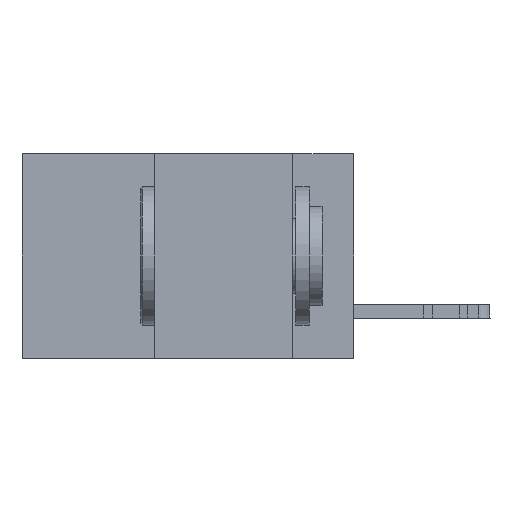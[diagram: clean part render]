
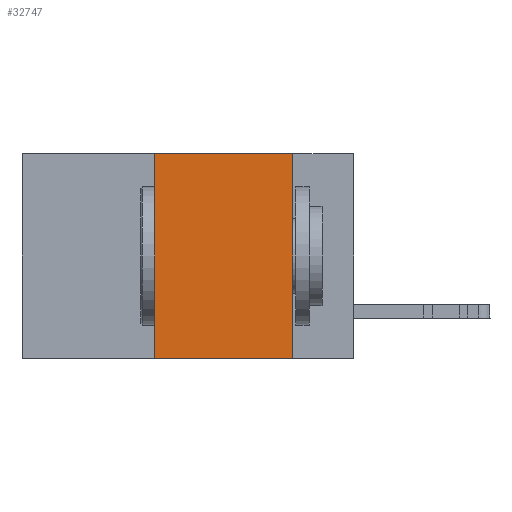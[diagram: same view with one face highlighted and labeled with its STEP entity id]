
A CAD part, left-side view. The second image highlights one B-rep face of the part: STEP entity #32747.
In plain terms, the highlighted planar face has unit normal (-1, 0, 0).
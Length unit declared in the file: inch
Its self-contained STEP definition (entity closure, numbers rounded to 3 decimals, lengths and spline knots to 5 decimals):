
#1204 = VERTEX_POINT ( 'NONE', #24172 ) ;
#1741 = VECTOR ( 'NONE', #41531, 39.37008 ) ;
#6698 = CARTESIAN_POINT ( 'NONE',  ( 0., 0.11, 0. ) ) ;
#12071 = LINE ( 'NONE', #14027, #20456 ) ;
#13984 = FACE_OUTER_BOUND ( 'NONE', #40193, .T. ) ;
#13990 = DIRECTION ( 'NONE',  ( 0., 0., -1. ) ) ;
#14027 = CARTESIAN_POINT ( 'NONE',  ( 0., 0.6, -0.37 ) ) ;
#15195 = VERTEX_POINT ( 'NONE', #22271 ) ;
#15994 = EDGE_CURVE ( 'NONE', #1204, #47161, #20562, .T. ) ;
#16484 = CARTESIAN_POINT ( 'NONE',  ( 0., 0.6, 0. ) ) ;
#17156 = EDGE_CURVE ( 'NONE', #47161, #15195, #27197, .T. ) ;
#18079 = VECTOR ( 'NONE', #13990, 39.37008 ) ;
#19020 = DIRECTION ( 'NONE',  ( 1., 0., 0. ) ) ;
#19328 = CARTESIAN_POINT ( 'NONE',  ( 0., 0.6, 0. ) ) ;
#20456 = VECTOR ( 'NONE', #33123, 39.37008 ) ;
#20562 = LINE ( 'NONE', #16484, #47250 ) ;
#20992 = CARTESIAN_POINT ( 'NONE',  ( 0., 0.11, 0. ) ) ;
#22271 = CARTESIAN_POINT ( 'NONE',  ( 0., 0.11, -0.37 ) ) ;
#23667 = PLANE ( 'NONE',  #24256 ) ;
#24110 = ORIENTED_EDGE ( 'NONE', *, *, #15994, .F. ) ;
#24172 = CARTESIAN_POINT ( 'NONE',  ( 0., 0.36, 0. ) ) ;
#24253 = CARTESIAN_POINT ( 'NONE',  ( 0., 0.36, -0.37 ) ) ;
#24256 = AXIS2_PLACEMENT_3D ( 'NONE', #19328, #19020, #30412 ) ;
#24885 = LINE ( 'NONE', #37453, #1741 ) ;
#25823 = ORIENTED_EDGE ( 'NONE', *, *, #27186, .T. ) ;
#26753 = VERTEX_POINT ( 'NONE', #24253 ) ;
#27186 = EDGE_CURVE ( 'NONE', #26753, #15195, #12071, .T. ) ;
#27197 = LINE ( 'NONE', #6698, #18079 ) ;
#27892 = ORIENTED_EDGE ( 'NONE', *, *, #46252, .F. ) ;
#30412 = DIRECTION ( 'NONE',  ( 0., 0., -1. ) ) ;
#32747 = ADVANCED_FACE ( 'NONE', ( #13984 ), #23667, .F. ) ;
#33123 = DIRECTION ( 'NONE',  ( 0., -1., 0. ) ) ;
#37453 = CARTESIAN_POINT ( 'NONE',  ( 0., 0.36, 0. ) ) ;
#40193 = EDGE_LOOP ( 'NONE', ( #49397, #24110, #27892, #25823 ) ) ;
#41531 = DIRECTION ( 'NONE',  ( 0., 0., 1. ) ) ;
#43512 = DIRECTION ( 'NONE',  ( 0., -1., 0. ) ) ;
#46252 = EDGE_CURVE ( 'NONE', #26753, #1204, #24885, .T. ) ;
#47161 = VERTEX_POINT ( 'NONE', #20992 ) ;
#47250 = VECTOR ( 'NONE', #43512, 39.37008 ) ;
#49397 = ORIENTED_EDGE ( 'NONE', *, *, #17156, .F. ) ;
